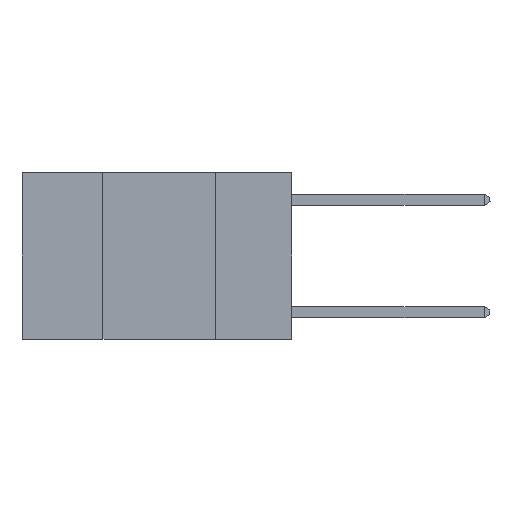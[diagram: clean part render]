
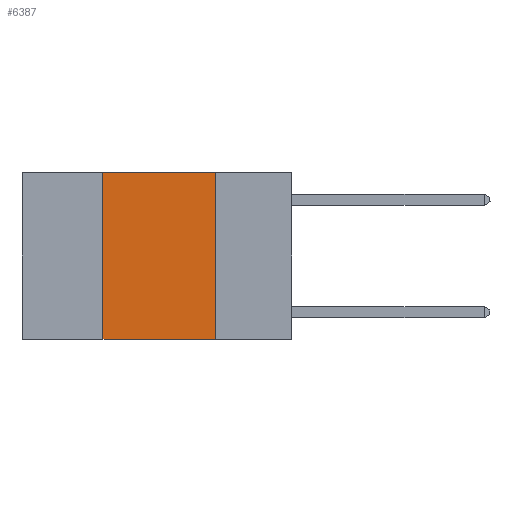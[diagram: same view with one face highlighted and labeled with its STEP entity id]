
A CAD part, left-side view. The second image highlights one B-rep face of the part: STEP entity #6387.
In plain terms, the highlighted planar face has unit normal (-1, 0, 0).
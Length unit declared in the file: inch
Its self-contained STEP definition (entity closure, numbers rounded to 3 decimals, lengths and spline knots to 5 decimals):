
#364 = EDGE_CURVE ( 'NONE', #5721, #7563, #4105, .T. ) ;
#500 = VECTOR ( 'NONE', #7725, 39.37008 ) ;
#824 = ORIENTED_EDGE ( 'NONE', *, *, #3980, .T. ) ;
#1115 = EDGE_CURVE ( 'NONE', #7563, #8445, #8308, .T. ) ;
#1240 = ORIENTED_EDGE ( 'NONE', *, *, #364, .F. ) ;
#1729 = DIRECTION ( 'NONE',  ( 0., -1., 0. ) ) ;
#1757 = ORIENTED_EDGE ( 'NONE', *, *, #1115, .F. ) ;
#2074 = VECTOR ( 'NONE', #6076, 39.37008 ) ;
#2097 = EDGE_LOOP ( 'NONE', ( #2339, #1757, #1240, #824 ) ) ;
#2116 = VERTEX_POINT ( 'NONE', #3430 ) ;
#2138 = EDGE_CURVE ( 'NONE', #8445, #2116, #6443, .T. ) ;
#2339 = ORIENTED_EDGE ( 'NONE', *, *, #2138, .F. ) ;
#2438 = VECTOR ( 'NONE', #2973, 39.37008 ) ;
#2973 = DIRECTION ( 'NONE',  ( 0., 0., -1. ) ) ;
#3089 = CARTESIAN_POINT ( 'NONE',  ( 0., 0.17, 0. ) ) ;
#3430 = CARTESIAN_POINT ( 'NONE',  ( 0., 0.17, -0.37 ) ) ;
#3499 = DIRECTION ( 'NONE',  ( 0., 0., -1. ) ) ;
#3921 = LINE ( 'NONE', #6289, #2074 ) ;
#3980 = EDGE_CURVE ( 'NONE', #5721, #2116, #3921, .T. ) ;
#4105 = LINE ( 'NONE', #7777, #500 ) ;
#5721 = VERTEX_POINT ( 'NONE', #7797 ) ;
#5805 = CARTESIAN_POINT ( 'NONE',  ( 0., 0.6, 0. ) ) ;
#6049 = CARTESIAN_POINT ( 'NONE',  ( 0., 0.42, 0. ) ) ;
#6076 = DIRECTION ( 'NONE',  ( 0., -1., 0. ) ) ;
#6107 = CARTESIAN_POINT ( 'NONE',  ( 0., 0.6, 0. ) ) ;
#6289 = CARTESIAN_POINT ( 'NONE',  ( 0., 0.6, -0.37 ) ) ;
#6387 = ADVANCED_FACE ( 'NONE', ( #7823 ), #7266, .F. ) ;
#6443 = LINE ( 'NONE', #3089, #2438 ) ;
#6797 = VECTOR ( 'NONE', #1729, 39.37008 ) ;
#7208 = CARTESIAN_POINT ( 'NONE',  ( 0., 0.17, 0. ) ) ;
#7266 = PLANE ( 'NONE',  #7272 ) ;
#7272 = AXIS2_PLACEMENT_3D ( 'NONE', #5805, #7924, #3499 ) ;
#7563 = VERTEX_POINT ( 'NONE', #6049 ) ;
#7725 = DIRECTION ( 'NONE',  ( 0., 0., 1. ) ) ;
#7777 = CARTESIAN_POINT ( 'NONE',  ( 0., 0.42, 0. ) ) ;
#7797 = CARTESIAN_POINT ( 'NONE',  ( 0., 0.42, -0.37 ) ) ;
#7823 = FACE_OUTER_BOUND ( 'NONE', #2097, .T. ) ;
#7924 = DIRECTION ( 'NONE',  ( 1., 0., 0. ) ) ;
#8308 = LINE ( 'NONE', #6107, #6797 ) ;
#8445 = VERTEX_POINT ( 'NONE', #7208 ) ;
